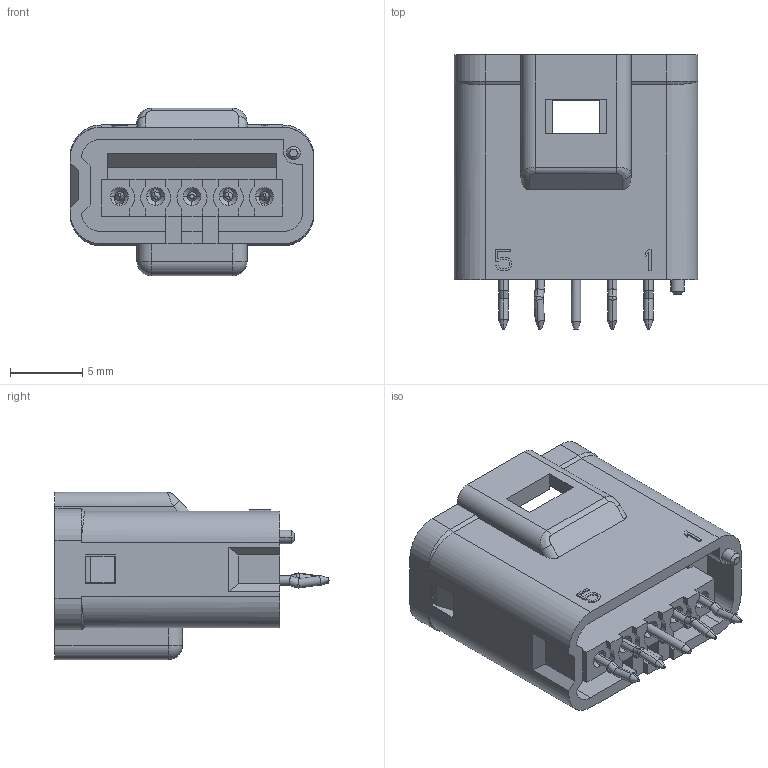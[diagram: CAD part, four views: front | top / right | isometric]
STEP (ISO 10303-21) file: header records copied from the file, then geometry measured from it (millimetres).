
FILE_DESCRIPTION (( 'STEP AP203' ), '1' );
FILE_NAME ('560-005-420-501.STEP', '2020-07-24T16:54:46', ( '' ), ( '' ), 'SwSTEP 2.0', 'SolidWorks 2020', '' );
FILE_SCHEMA (( 'CONFIG_CONTROL_DESIGN' ));
Length unit declared in the file: millimetre
Products named in the file (10): CONTACT_PCB-HEADER-2; CONTACT_PCB-HEADER-1; 560-005-420-501; CONTACT_PCB-HEADER; FACIAL_SEAL_5POS; PCB-HEADER-CONTACT-5P; CONTACT_PCB-HEADER-3; INTERNAL-WIRE-SEAL-5POS; PCB-HEADER-HOUSING-5P_ORANGE
Assembly tree (9 placements, depth 3):
  560-005-420-501
    560-005-420-501
      PCB-HEADER-HOUSING-5P_ORANGE
      CONTACT_PCB-HEADER
      CONTACT_PCB-HEADER-1
      PCB-HEADER-CONTACT-5P
      CONTACT_PCB-HEADER-2
      CONTACT_PCB-HEADER-3
      INTERNAL-WIRE-SEAL-5POS
      FACIAL_SEAL_5POS
Bounding box: 16.8 x 18.9 x 11.55 mm (x, y, z)
Volume: 1028.4 mm3; surface area: 2868.8 mm2
Topology: 8 solids, 8 shells, 772 faces, 1933 edges, 1198 vertices
Faces by surface type: plane 448, cylinder 184, cone 84, torus 44, bspline 10, sphere 2
Entity records: 24563 total; most frequent: CARTESIAN_POINT 5032, ORIENTED_EDGE 3862, DIRECTION 3831, EDGE_CURVE 1931, VECTOR 1289, LINE 1289, AXIS2_PLACEMENT_3D 1271, VERTEX_POINT 1198
